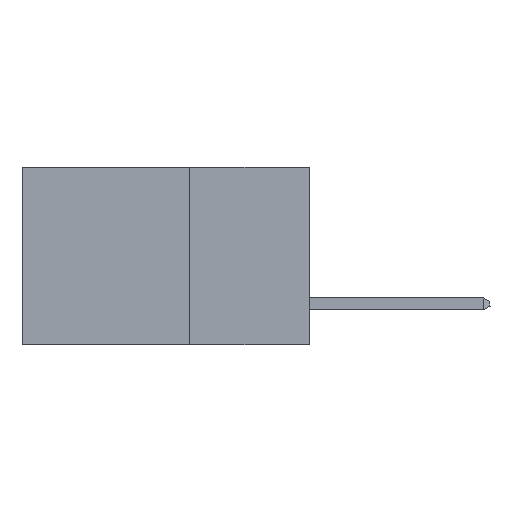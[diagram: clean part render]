
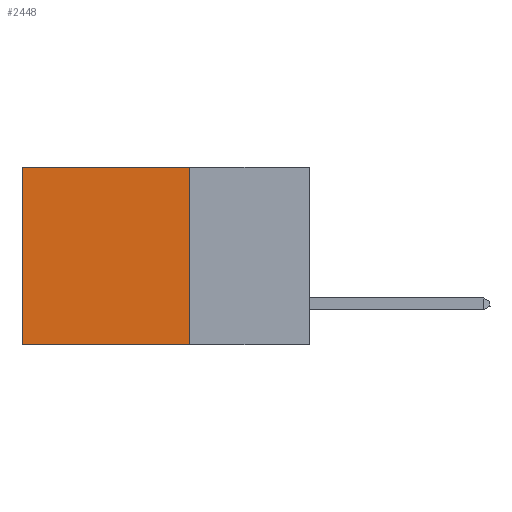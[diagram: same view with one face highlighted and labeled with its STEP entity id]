
A CAD part, left-side view. The second image highlights one B-rep face of the part: STEP entity #2448.
In plain terms, the highlighted planar face has unit normal (-1, 0, 0).
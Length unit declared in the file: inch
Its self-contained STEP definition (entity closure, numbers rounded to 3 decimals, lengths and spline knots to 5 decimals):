
#221 = PLANE ( 'NONE',  #11285 ) ;
#631 = ORIENTED_EDGE ( 'NONE', *, *, #3693, .F. ) ;
#1909 = DIRECTION ( 'NONE',  ( 1., 0., 0. ) ) ;
#2448 = ADVANCED_FACE ( 'NONE', ( #22879 ), #221, .F. ) ;
#3006 = ORIENTED_EDGE ( 'NONE', *, *, #21649, .F. ) ;
#3245 = VERTEX_POINT ( 'NONE', #9869 ) ;
#3287 = CARTESIAN_POINT ( 'NONE',  ( 0.2875, 0.25, 0. ) ) ;
#3693 = EDGE_CURVE ( 'NONE', #3245, #19214, #21728, .T. ) ;
#4236 = EDGE_CURVE ( 'NONE', #3245, #15360, #6021, .T. ) ;
#6021 = LINE ( 'NONE', #3287, #18516 ) ;
#7131 = DIRECTION ( 'NONE',  ( 0., 1., 0. ) ) ;
#7760 = CARTESIAN_POINT ( 'NONE',  ( 0.2875, 0.6, 0. ) ) ;
#9064 = CARTESIAN_POINT ( 'NONE',  ( 0.2875, 0.25, -0.37 ) ) ;
#9401 = EDGE_LOOP ( 'NONE', ( #22535, #3006, #631, #15962 ) ) ;
#9774 = CARTESIAN_POINT ( 'NONE',  ( 0.2875, 0.6, 0. ) ) ;
#9869 = CARTESIAN_POINT ( 'NONE',  ( 0.2875, 0.25, 0. ) ) ;
#10454 = LINE ( 'NONE', #9774, #21245 ) ;
#10871 = DIRECTION ( 'NONE',  ( 0., 0., -1. ) ) ;
#11285 = AXIS2_PLACEMENT_3D ( 'NONE', #14763, #1909, #10871 ) ;
#11328 = EDGE_CURVE ( 'NONE', #15360, #18274, #10454, .T. ) ;
#13628 = DIRECTION ( 'NONE',  ( 0., 0., -1. ) ) ;
#14763 = CARTESIAN_POINT ( 'NONE',  ( 0.2875, 0.25, 0. ) ) ;
#15360 = VERTEX_POINT ( 'NONE', #7760 ) ;
#15442 = CARTESIAN_POINT ( 'NONE',  ( 0.2875, 0.25, 0. ) ) ;
#15962 = ORIENTED_EDGE ( 'NONE', *, *, #4236, .T. ) ;
#15991 = DIRECTION ( 'NONE',  ( 0., 1., 0. ) ) ;
#16997 = DIRECTION ( 'NONE',  ( 0., 0., -1. ) ) ;
#17089 = VECTOR ( 'NONE', #7131, 39.37008 ) ;
#17463 = VECTOR ( 'NONE', #13628, 39.37008 ) ;
#18274 = VERTEX_POINT ( 'NONE', #20976 ) ;
#18516 = VECTOR ( 'NONE', #15991, 39.37008 ) ;
#19031 = CARTESIAN_POINT ( 'NONE',  ( 0.2875, 0.25, -0.37 ) ) ;
#19214 = VERTEX_POINT ( 'NONE', #9064 ) ;
#20477 = LINE ( 'NONE', #19031, #17089 ) ;
#20976 = CARTESIAN_POINT ( 'NONE',  ( 0.2875, 0.6, -0.37 ) ) ;
#21245 = VECTOR ( 'NONE', #16997, 39.37008 ) ;
#21649 = EDGE_CURVE ( 'NONE', #19214, #18274, #20477, .T. ) ;
#21728 = LINE ( 'NONE', #15442, #17463 ) ;
#22535 = ORIENTED_EDGE ( 'NONE', *, *, #11328, .T. ) ;
#22879 = FACE_OUTER_BOUND ( 'NONE', #9401, .T. ) ;
